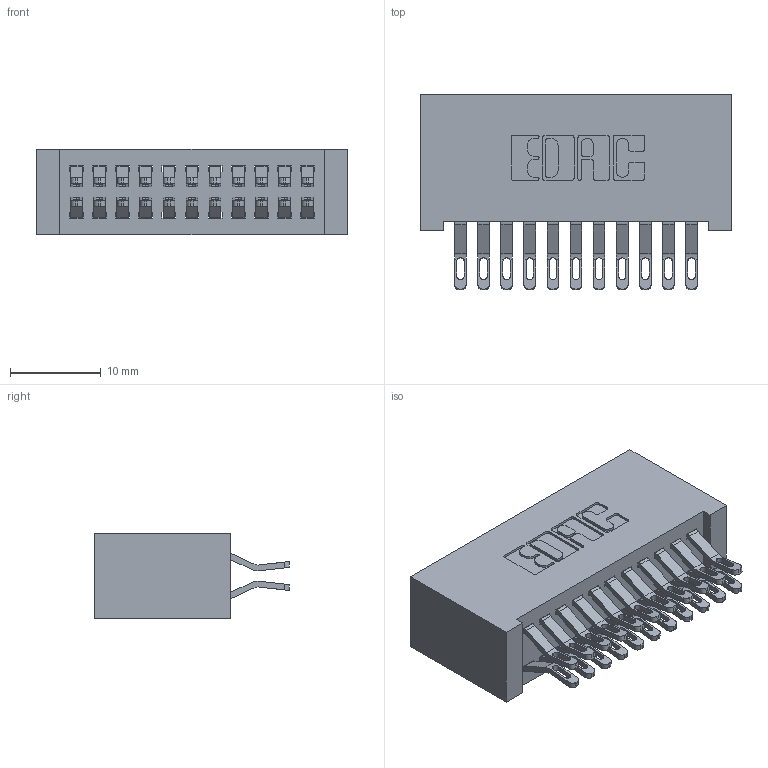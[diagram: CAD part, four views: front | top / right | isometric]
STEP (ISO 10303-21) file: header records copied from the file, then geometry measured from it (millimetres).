
FILE_DESCRIPTION (( 'STEP AP203' ), '1' );
FILE_NAME ('392-022-555-201.STEP', '2019-10-07T06:28:11', ( '' ), ( '' ), 'SwSTEP 2.0', 'SolidWorks 2016', '' );
FILE_SCHEMA (( 'CONFIG_CONTROL_DESIGN' ));
Length unit declared in the file: inch
Products named in the file (3): 342 Part_Lugless; 345-292-001_555 Tail; 392-022-555-201
Assembly tree (23 placements, depth 2):
  392-022-555-201
    342 Part_Lugless
    345-292-001_555 Tail  x22
Bounding box: 34.19 x 21.47 x 9.4 mm (x, y, z)
Volume: 3425.7 mm3; surface area: 5471.5 mm2
Topology: 23 solids, 23 shells, 1378 faces, 4301 edges, 2866 vertices
Faces by surface type: plane 810, cylinder 568
Entity records: 11003 total; most frequent: CARTESIAN_POINT 1892, ORIENTED_EDGE 1798, DIRECTION 1635, EDGE_CURVE 899, LINE 759, VECTOR 759, VERTEX_POINT 598, AXIS2_PLACEMENT_3D 438
